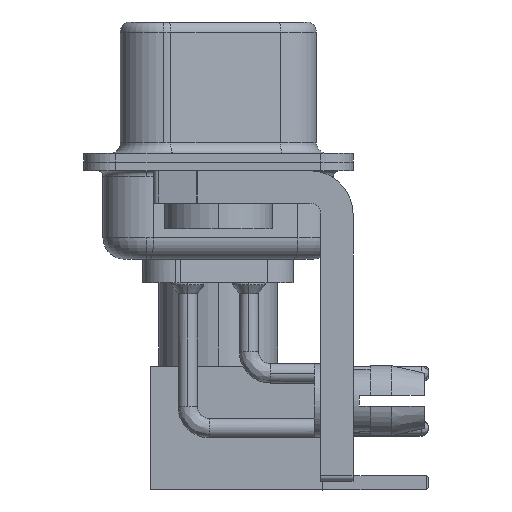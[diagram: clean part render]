
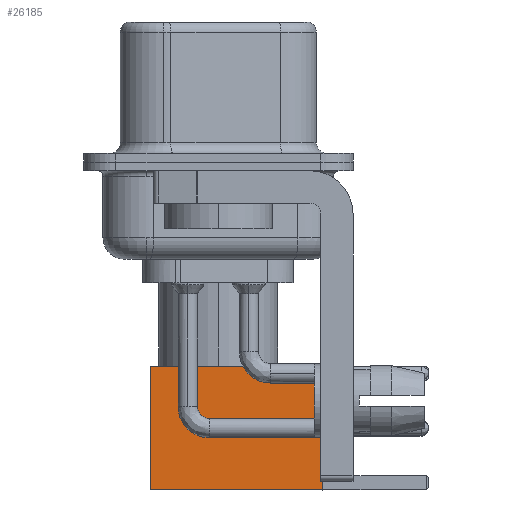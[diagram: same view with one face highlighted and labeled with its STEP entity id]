
A CAD part, left-side view. The second image highlights one B-rep face of the part: STEP entity #26185.
In plain terms, the highlighted face is planar.
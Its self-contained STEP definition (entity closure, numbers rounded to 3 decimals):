
#965 = DIRECTION ( 'NONE',  ( 0., 0., -1. ) ) ;
#1766 = VECTOR ( 'NONE', #19146, 1000. ) ;
#3312 = CARTESIAN_POINT ( 'NONE',  ( -2.875, 2.875, 0. ) ) ;
#3883 = VERTEX_POINT ( 'NONE', #16149 ) ;
#4186 = EDGE_CURVE ( 'NONE', #3883, #10739, #26099, .T. ) ;
#4655 = VERTEX_POINT ( 'NONE', #26922 ) ;
#5620 = VECTOR ( 'NONE', #15122, 1000. ) ;
#6193 = CARTESIAN_POINT ( 'NONE',  ( 0., 2.875, 0. ) ) ;
#8980 = PLANE ( 'NONE',  #25835 ) ;
#9531 = CARTESIAN_POINT ( 'NONE',  ( 0., 2.875, 8. ) ) ;
#10226 = EDGE_LOOP ( 'NONE', ( #12060, #17735, #14112, #19994 ) ) ;
#10739 = VERTEX_POINT ( 'NONE', #14014 ) ;
#11045 = VERTEX_POINT ( 'NONE', #26876 ) ;
#11716 = LINE ( 'NONE', #9531, #16527 ) ;
#11746 = FACE_OUTER_BOUND ( 'NONE', #10226, .T. ) ;
#12060 = ORIENTED_EDGE ( 'NONE', *, *, #16778, .T. ) ;
#14014 = CARTESIAN_POINT ( 'NONE',  ( -2.875, 2.875, 0. ) ) ;
#14112 = ORIENTED_EDGE ( 'NONE', *, *, #24582, .F. ) ;
#15122 = DIRECTION ( 'NONE',  ( -1., 0., 0. ) ) ;
#16117 = DIRECTION ( 'NONE',  ( -1., 0., 0. ) ) ;
#16149 = CARTESIAN_POINT ( 'NONE',  ( 2.875, 2.875, 0. ) ) ;
#16527 = VECTOR ( 'NONE', #16117, 1000. ) ;
#16778 = EDGE_CURVE ( 'NONE', #11045, #3883, #25877, .T. ) ;
#16799 = CARTESIAN_POINT ( 'NONE',  ( 2.875, 2.875, 0. ) ) ;
#17735 = ORIENTED_EDGE ( 'NONE', *, *, #4186, .T. ) ;
#18340 = CARTESIAN_POINT ( 'NONE',  ( 2.875, 2.875, 0. ) ) ;
#19146 = DIRECTION ( 'NONE',  ( 0., 0., -1. ) ) ;
#19994 = ORIENTED_EDGE ( 'NONE', *, *, #28862, .F. ) ;
#20686 = DIRECTION ( 'NONE',  ( 0., 1., 0. ) ) ;
#21156 = LINE ( 'NONE', #3312, #21756 ) ;
#21756 = VECTOR ( 'NONE', #965, 1000. ) ;
#24582 = EDGE_CURVE ( 'NONE', #4655, #10739, #21156, .T. ) ;
#24933 = DIRECTION ( 'NONE',  ( 0., 0., 1. ) ) ;
#25835 = AXIS2_PLACEMENT_3D ( 'NONE', #18340, #20686, #24933 ) ;
#25877 = LINE ( 'NONE', #16799, #1766 ) ;
#26099 = LINE ( 'NONE', #6193, #5620 ) ;
#26185 = ADVANCED_FACE ( 'NONE', ( #11746 ), #8980, .T. ) ;
#26876 = CARTESIAN_POINT ( 'NONE',  ( 2.875, 2.875, 8. ) ) ;
#26922 = CARTESIAN_POINT ( 'NONE',  ( -2.875, 2.875, 8. ) ) ;
#28862 = EDGE_CURVE ( 'NONE', #11045, #4655, #11716, .T. ) ;
